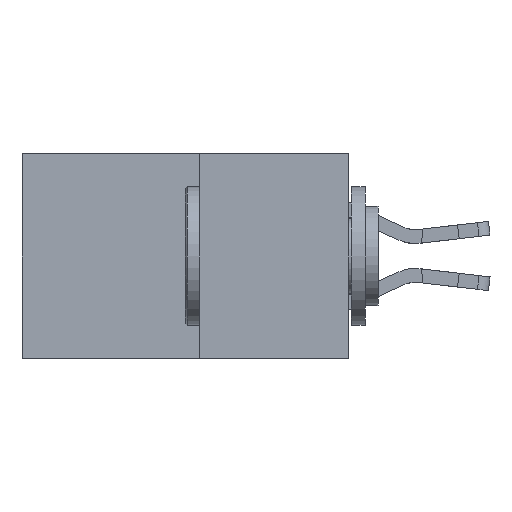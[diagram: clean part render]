
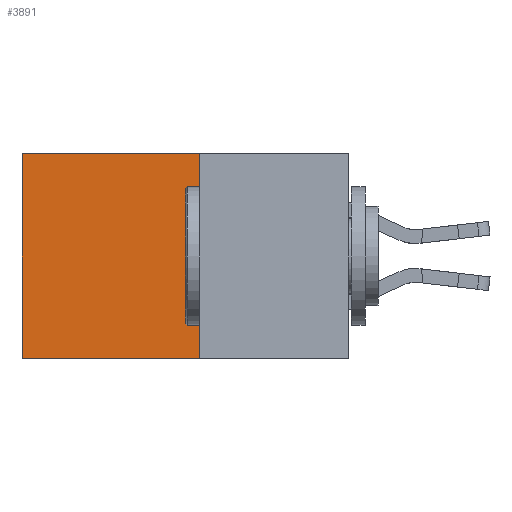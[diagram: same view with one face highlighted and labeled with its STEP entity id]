
A CAD part, left-side view. The second image highlights one B-rep face of the part: STEP entity #3891.
In plain terms, the highlighted planar face has unit normal (-1, 0, 0).
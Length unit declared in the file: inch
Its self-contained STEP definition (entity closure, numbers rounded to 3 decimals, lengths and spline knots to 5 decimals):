
#182 = ORIENTED_EDGE ( 'NONE', *, *, #5904, .T. ) ;
#2238 = DIRECTION ( 'NONE',  ( 0., 0., -1. ) ) ;
#2272 = CARTESIAN_POINT ( 'NONE',  ( 0.277, 0.59, -0.37 ) ) ;
#3318 = CARTESIAN_POINT ( 'NONE',  ( 0.277, 0.27, -0.37 ) ) ;
#3437 = DIRECTION ( 'NONE',  ( 0., 0., -1. ) ) ;
#3628 = CARTESIAN_POINT ( 'NONE',  ( 0.277, 0.27, 0. ) ) ;
#3860 = CARTESIAN_POINT ( 'NONE',  ( 0.277, 0.27, -0.37 ) ) ;
#3891 = ADVANCED_FACE ( 'NONE', ( #24309 ), #25183, .F. ) ;
#4144 = DIRECTION ( 'NONE',  ( 0., 1., 0. ) ) ;
#4389 = EDGE_CURVE ( 'NONE', #18824, #10833, #11948, .T. ) ;
#5469 = CARTESIAN_POINT ( 'NONE',  ( 0.277, 0.59, 0. ) ) ;
#5904 = EDGE_CURVE ( 'NONE', #13439, #10833, #7234, .T. ) ;
#6341 = VECTOR ( 'NONE', #20417, 39.37008 ) ;
#7234 = LINE ( 'NONE', #2272, #18323 ) ;
#7661 = EDGE_CURVE ( 'NONE', #8457, #18824, #21440, .T. ) ;
#8186 = ORIENTED_EDGE ( 'NONE', *, *, #7661, .F. ) ;
#8457 = VERTEX_POINT ( 'NONE', #11204 ) ;
#9809 = EDGE_CURVE ( 'NONE', #8457, #13439, #13976, .T. ) ;
#10833 = VERTEX_POINT ( 'NONE', #24033 ) ;
#11204 = CARTESIAN_POINT ( 'NONE',  ( 0.277, 0.27, 0. ) ) ;
#11948 = LINE ( 'NONE', #20714, #6341 ) ;
#13439 = VERTEX_POINT ( 'NONE', #5469 ) ;
#13976 = LINE ( 'NONE', #3628, #25004 ) ;
#14913 = AXIS2_PLACEMENT_3D ( 'NONE', #24154, #23484, #24541 ) ;
#15219 = EDGE_LOOP ( 'NONE', ( #182, #18798, #8186, #20418 ) ) ;
#18323 = VECTOR ( 'NONE', #2238, 39.37008 ) ;
#18798 = ORIENTED_EDGE ( 'NONE', *, *, #4389, .F. ) ;
#18824 = VERTEX_POINT ( 'NONE', #3860 ) ;
#20417 = DIRECTION ( 'NONE',  ( 0., 1., 0. ) ) ;
#20418 = ORIENTED_EDGE ( 'NONE', *, *, #9809, .T. ) ;
#20714 = CARTESIAN_POINT ( 'NONE',  ( 0.277, 0.27, -0.37 ) ) ;
#21440 = LINE ( 'NONE', #3318, #26370 ) ;
#23484 = DIRECTION ( 'NONE',  ( 1., 0., 0. ) ) ;
#24033 = CARTESIAN_POINT ( 'NONE',  ( 0.277, 0.59, -0.37 ) ) ;
#24154 = CARTESIAN_POINT ( 'NONE',  ( 0.277, 0.27, -0.37 ) ) ;
#24309 = FACE_OUTER_BOUND ( 'NONE', #15219, .T. ) ;
#24541 = DIRECTION ( 'NONE',  ( 0., 0., -1. ) ) ;
#25004 = VECTOR ( 'NONE', #4144, 39.37008 ) ;
#25183 = PLANE ( 'NONE',  #14913 ) ;
#26370 = VECTOR ( 'NONE', #3437, 39.37008 ) ;
